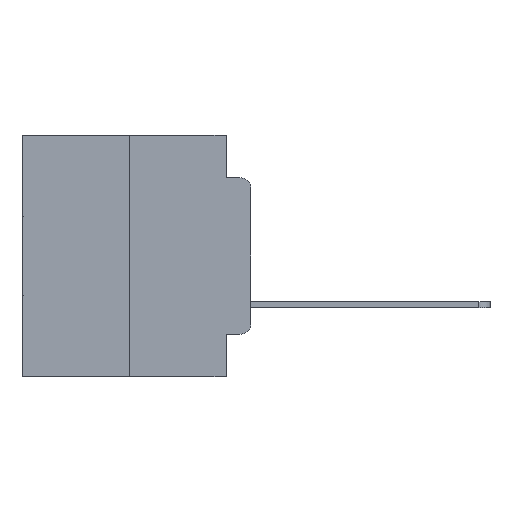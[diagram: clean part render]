
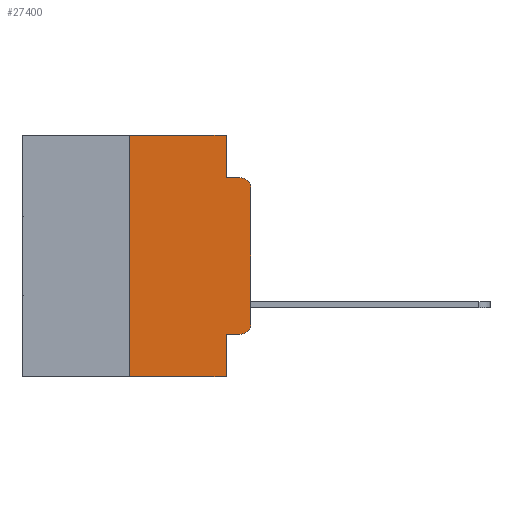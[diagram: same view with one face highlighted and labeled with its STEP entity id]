
A CAD part, left-side view. The second image highlights one B-rep face of the part: STEP entity #27400.
In plain terms, the highlighted planar face has unit normal (-1, 0, 0).
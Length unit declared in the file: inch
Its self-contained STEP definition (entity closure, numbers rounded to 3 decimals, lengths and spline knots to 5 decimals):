
#509 = EDGE_CURVE ( 'NONE', #3547, #10532, #15367, .T. ) ;
#526 = VECTOR ( 'NONE', #26196, 39.37008 ) ;
#921 = CARTESIAN_POINT ( 'NONE',  ( 0., 0.051, -0.5 ) ) ;
#1059 = CARTESIAN_POINT ( 'NONE',  ( 0., 0.25, 0. ) ) ;
#1098 = EDGE_CURVE ( 'NONE', #2712, #16582, #28275, .T. ) ;
#1424 = LINE ( 'NONE', #11809, #18562 ) ;
#2259 = PLANE ( 'NONE',  #19773 ) ;
#2367 = DIRECTION ( 'NONE',  ( 0., 0., -1. ) ) ;
#2712 = VERTEX_POINT ( 'NONE', #6175 ) ;
#3475 = ORIENTED_EDGE ( 'NONE', *, *, #7195, .F. ) ;
#3547 = VERTEX_POINT ( 'NONE', #6068 ) ;
#3667 = CARTESIAN_POINT ( 'NONE',  ( 0., 0.051, 0. ) ) ;
#3856 = DIRECTION ( 'NONE',  ( -1., 0., 0. ) ) ;
#3863 = DIRECTION ( 'NONE',  ( 0., 0., -1. ) ) ;
#3888 = CARTESIAN_POINT ( 'NONE',  ( 0., 0.02, -0.1085 ) ) ;
#4179 = EDGE_LOOP ( 'NONE', ( #15403, #21034, #20175, #26438, #4746, #3475, #9971, #5715, #17752, #4980 ) ) ;
#4251 = EDGE_CURVE ( 'NONE', #26860, #10532, #20559, .T. ) ;
#4529 = FACE_OUTER_BOUND ( 'NONE', #4179, .T. ) ;
#4746 = ORIENTED_EDGE ( 'NONE', *, *, #22743, .F. ) ;
#4860 = DIRECTION ( 'NONE',  ( 0., -1., 0. ) ) ;
#4980 = ORIENTED_EDGE ( 'NONE', *, *, #1098, .T. ) ;
#5147 = VECTOR ( 'NONE', #12326, 39.37008 ) ;
#5715 = ORIENTED_EDGE ( 'NONE', *, *, #17590, .F. ) ;
#5725 = EDGE_CURVE ( 'NONE', #13428, #13754, #7643, .T. ) ;
#5774 = CARTESIAN_POINT ( 'NONE',  ( 0., 0.051, -0.4115 ) ) ;
#6050 = LINE ( 'NONE', #28172, #526 ) ;
#6068 = CARTESIAN_POINT ( 'NONE',  ( 0., 0., -0.1085 ) ) ;
#6175 = CARTESIAN_POINT ( 'NONE',  ( 0., 0.02, -0.4115 ) ) ;
#7195 = EDGE_CURVE ( 'NONE', #13428, #9031, #23850, .T. ) ;
#7643 = LINE ( 'NONE', #18088, #18577 ) ;
#8847 = CARTESIAN_POINT ( 'NONE',  ( 0., 0.25, -0.5 ) ) ;
#8924 = CARTESIAN_POINT ( 'NONE',  ( 0., 0.02, -0.3915 ) ) ;
#9031 = VERTEX_POINT ( 'NONE', #21240 ) ;
#9514 = CARTESIAN_POINT ( 'NONE',  ( 0., 0.051, -0.0885 ) ) ;
#9737 = VECTOR ( 'NONE', #23369, 39.37008 ) ;
#9971 = ORIENTED_EDGE ( 'NONE', *, *, #5725, .T. ) ;
#10441 = LINE ( 'NONE', #27289, #5147 ) ;
#10532 = VERTEX_POINT ( 'NONE', #17670 ) ;
#10689 = EDGE_CURVE ( 'NONE', #24850, #2712, #1424, .T. ) ;
#11099 = CARTESIAN_POINT ( 'NONE',  ( 0., 0.473, 0. ) ) ;
#11809 = CARTESIAN_POINT ( 'NONE',  ( 0., 0.051, -0.4115 ) ) ;
#11973 = CARTESIAN_POINT ( 'NONE',  ( 0., 0., -0.3915 ) ) ;
#12326 = DIRECTION ( 'NONE',  ( 0., 0., -1. ) ) ;
#12692 = VERTEX_POINT ( 'NONE', #3667 ) ;
#13428 = VERTEX_POINT ( 'NONE', #8847 ) ;
#13684 = CARTESIAN_POINT ( 'NONE',  ( 0., 0.473, 0. ) ) ;
#13754 = VERTEX_POINT ( 'NONE', #921 ) ;
#15367 = CIRCLE ( 'NONE', #24014, 0.02 ) ;
#15403 = ORIENTED_EDGE ( 'NONE', *, *, #25099, .T. ) ;
#15573 = LINE ( 'NONE', #21202, #9737 ) ;
#15637 = VECTOR ( 'NONE', #17640, 39.37008 ) ;
#15766 = AXIS2_PLACEMENT_3D ( 'NONE', #8924, #26479, #27071 ) ;
#15885 = DIRECTION ( 'NONE',  ( 1., 0., 0. ) ) ;
#16582 = VERTEX_POINT ( 'NONE', #11973 ) ;
#16788 = EDGE_CURVE ( 'NONE', #12692, #26860, #15573, .T. ) ;
#17590 = EDGE_CURVE ( 'NONE', #24850, #13754, #10441, .T. ) ;
#17640 = DIRECTION ( 'NONE',  ( 0., -1., 0. ) ) ;
#17670 = CARTESIAN_POINT ( 'NONE',  ( 0., 0.02, -0.0885 ) ) ;
#17752 = ORIENTED_EDGE ( 'NONE', *, *, #10689, .T. ) ;
#18088 = CARTESIAN_POINT ( 'NONE',  ( 0., 0.473, -0.5 ) ) ;
#18125 = VECTOR ( 'NONE', #21114, 39.37008 ) ;
#18562 = VECTOR ( 'NONE', #22569, 39.37008 ) ;
#18577 = VECTOR ( 'NONE', #4860, 39.37008 ) ;
#19773 = AXIS2_PLACEMENT_3D ( 'NONE', #13684, #15885, #2367 ) ;
#20175 = ORIENTED_EDGE ( 'NONE', *, *, #4251, .F. ) ;
#20559 = LINE ( 'NONE', #9514, #24918 ) ;
#21034 = ORIENTED_EDGE ( 'NONE', *, *, #509, .T. ) ;
#21114 = DIRECTION ( 'NONE',  ( 0., 0., 1. ) ) ;
#21202 = CARTESIAN_POINT ( 'NONE',  ( 0., 0.051, 0. ) ) ;
#21240 = CARTESIAN_POINT ( 'NONE',  ( 0., 0.25, 0. ) ) ;
#21343 = LINE ( 'NONE', #11099, #15637 ) ;
#22566 = CARTESIAN_POINT ( 'NONE',  ( 0., 0.051, -0.0885 ) ) ;
#22569 = DIRECTION ( 'NONE',  ( 0., -1., 0. ) ) ;
#22743 = EDGE_CURVE ( 'NONE', #9031, #12692, #21343, .T. ) ;
#22853 = DIRECTION ( 'NONE',  ( 0., -1., 0. ) ) ;
#23369 = DIRECTION ( 'NONE',  ( 0., 0., -1. ) ) ;
#23850 = LINE ( 'NONE', #1059, #18125 ) ;
#24014 = AXIS2_PLACEMENT_3D ( 'NONE', #3888, #3856, #3863 ) ;
#24850 = VERTEX_POINT ( 'NONE', #5774 ) ;
#24918 = VECTOR ( 'NONE', #22853, 39.37008 ) ;
#25099 = EDGE_CURVE ( 'NONE', #16582, #3547, #6050, .T. ) ;
#26196 = DIRECTION ( 'NONE',  ( 0., 0., 1. ) ) ;
#26438 = ORIENTED_EDGE ( 'NONE', *, *, #16788, .F. ) ;
#26479 = DIRECTION ( 'NONE',  ( -1., 0., 0. ) ) ;
#26860 = VERTEX_POINT ( 'NONE', #22566 ) ;
#27071 = DIRECTION ( 'NONE',  ( 0., 0., -1. ) ) ;
#27289 = CARTESIAN_POINT ( 'NONE',  ( 0., 0.051, 0. ) ) ;
#27400 = ADVANCED_FACE ( 'NONE', ( #4529 ), #2259, .F. ) ;
#28172 = CARTESIAN_POINT ( 'NONE',  ( 0., 0., 0. ) ) ;
#28275 = CIRCLE ( 'NONE', #15766, 0.02 ) ;
